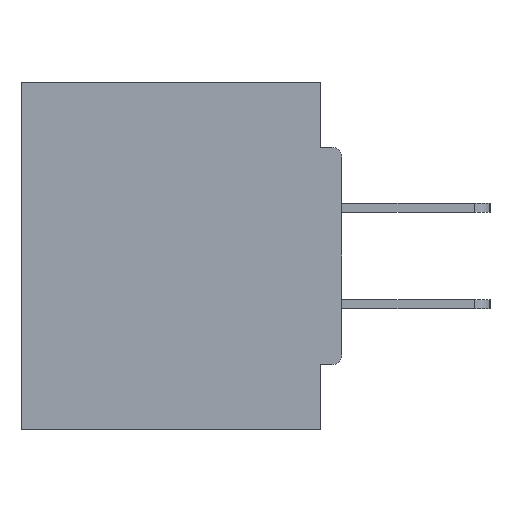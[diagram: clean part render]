
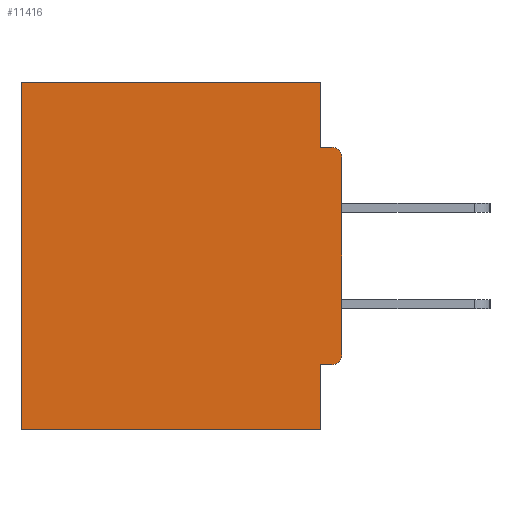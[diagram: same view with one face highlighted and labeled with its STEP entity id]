
A CAD part, left-side view. The second image highlights one B-rep face of the part: STEP entity #11416.
In plain terms, the highlighted planar face has unit normal (-1, 0, 0).
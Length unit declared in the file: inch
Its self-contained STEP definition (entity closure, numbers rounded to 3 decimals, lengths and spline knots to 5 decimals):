
#452 = DIRECTION ( 'NONE',  ( -1., 0., 0. ) ) ;
#820 = CARTESIAN_POINT ( 'NONE',  ( 0.298, 0.031, -0.4065 ) ) ;
#988 = DIRECTION ( 'NONE',  ( 0., 0., -1. ) ) ;
#1395 = AXIS2_PLACEMENT_3D ( 'NONE', #8110, #39183, #17584 ) ;
#1457 = VECTOR ( 'NONE', #15392, 39.37008 ) ;
#1541 = CARTESIAN_POINT ( 'NONE',  ( 0.298, 0.015, -0.4065 ) ) ;
#2151 = DIRECTION ( 'NONE',  ( 0., 0., -1. ) ) ;
#2194 = VERTEX_POINT ( 'NONE', #28801 ) ;
#2297 = LINE ( 'NONE', #12856, #6723 ) ;
#2359 = ORIENTED_EDGE ( 'NONE', *, *, #25466, .F. ) ;
#4178 = DIRECTION ( 'NONE',  ( 0., -1., 0. ) ) ;
#4212 = DIRECTION ( 'NONE',  ( 0., 0., -1. ) ) ;
#4924 = VECTOR ( 'NONE', #21846, 39.37008 ) ;
#5265 = ORIENTED_EDGE ( 'NONE', *, *, #29698, .T. ) ;
#5344 = CARTESIAN_POINT ( 'NONE',  ( 0.298, 0.031, 0. ) ) ;
#6353 = VERTEX_POINT ( 'NONE', #1541 ) ;
#6672 = VERTEX_POINT ( 'NONE', #12775 ) ;
#6723 = VECTOR ( 'NONE', #15697, 39.37008 ) ;
#6793 = LINE ( 'NONE', #25737, #36395 ) ;
#7207 = LINE ( 'NONE', #35267, #36298 ) ;
#7228 = EDGE_CURVE ( 'NONE', #10068, #6672, #9924, .T. ) ;
#8110 = CARTESIAN_POINT ( 'NONE',  ( 0.298, 0., 0. ) ) ;
#8902 = CARTESIAN_POINT ( 'NONE',  ( 0.298, 0., -0.5 ) ) ;
#8995 = EDGE_CURVE ( 'NONE', #6353, #25177, #26716, .T. ) ;
#9034 = DIRECTION ( 'NONE',  ( 0., 1., 0. ) ) ;
#9660 = CARTESIAN_POINT ( 'NONE',  ( 0.298, 0.031, -0.0935 ) ) ;
#9924 = LINE ( 'NONE', #25129, #39048 ) ;
#10068 = VERTEX_POINT ( 'NONE', #5344 ) ;
#10273 = CARTESIAN_POINT ( 'NONE',  ( 0.298, 0.015, -0.0935 ) ) ;
#10296 = VERTEX_POINT ( 'NONE', #820 ) ;
#10575 = CARTESIAN_POINT ( 'NONE',  ( 0.298, 0., -0.0935 ) ) ;
#11249 = VERTEX_POINT ( 'NONE', #35644 ) ;
#11416 = ADVANCED_FACE ( 'NONE', ( #39163 ), #29515, .F. ) ;
#12499 = CARTESIAN_POINT ( 'NONE',  ( 0.298, 0., 0. ) ) ;
#12775 = CARTESIAN_POINT ( 'NONE',  ( 0.298, 0.46, 0. ) ) ;
#12856 = CARTESIAN_POINT ( 'NONE',  ( 0.298, 0.031, -0.5 ) ) ;
#12966 = CARTESIAN_POINT ( 'NONE',  ( 0.298, 0.015, -0.3915 ) ) ;
#14225 = ORIENTED_EDGE ( 'NONE', *, *, #31308, .F. ) ;
#14509 = ORIENTED_EDGE ( 'NONE', *, *, #17757, .T. ) ;
#15040 = AXIS2_PLACEMENT_3D ( 'NONE', #30118, #33090, #2151 ) ;
#15070 = LINE ( 'NONE', #27434, #1457 ) ;
#15392 = DIRECTION ( 'NONE',  ( 0., 1., 0. ) ) ;
#15697 = DIRECTION ( 'NONE',  ( 0., 0., -1. ) ) ;
#16772 = ORIENTED_EDGE ( 'NONE', *, *, #24386, .F. ) ;
#16937 = LINE ( 'NONE', #8902, #22774 ) ;
#17584 = DIRECTION ( 'NONE',  ( 0., 0., -1. ) ) ;
#17757 = EDGE_CURVE ( 'NONE', #6672, #36067, #7207, .T. ) ;
#18346 = VERTEX_POINT ( 'NONE', #10273 ) ;
#21399 = LINE ( 'NONE', #12499, #4924 ) ;
#21846 = DIRECTION ( 'NONE',  ( 0., 0., -1. ) ) ;
#22373 = DIRECTION ( 'NONE',  ( 0., 0., -1. ) ) ;
#22774 = VECTOR ( 'NONE', #9034, 39.37008 ) ;
#22905 = CIRCLE ( 'NONE', #15040, 0.015 ) ;
#23426 = CARTESIAN_POINT ( 'NONE',  ( 0.298, 0., -0.3915 ) ) ;
#24315 = VERTEX_POINT ( 'NONE', #9660 ) ;
#24386 = EDGE_CURVE ( 'NONE', #11249, #25177, #21399, .T. ) ;
#25039 = ORIENTED_EDGE ( 'NONE', *, *, #36988, .F. ) ;
#25129 = CARTESIAN_POINT ( 'NONE',  ( 0.298, 0., 0. ) ) ;
#25177 = VERTEX_POINT ( 'NONE', #23426 ) ;
#25466 = EDGE_CURVE ( 'NONE', #2194, #36067, #16937, .T. ) ;
#25737 = CARTESIAN_POINT ( 'NONE',  ( 0.298, 0.031, -0.5 ) ) ;
#26505 = AXIS2_PLACEMENT_3D ( 'NONE', #12966, #452, #988 ) ;
#26621 = CARTESIAN_POINT ( 'NONE',  ( 0.298, 0.46, -0.5 ) ) ;
#26716 = CIRCLE ( 'NONE', #26505, 0.015 ) ;
#27434 = CARTESIAN_POINT ( 'NONE',  ( 0.298, 0., -0.4065 ) ) ;
#28212 = ORIENTED_EDGE ( 'NONE', *, *, #34033, .F. ) ;
#28801 = CARTESIAN_POINT ( 'NONE',  ( 0.298, 0.031, -0.5 ) ) ;
#29515 = PLANE ( 'NONE',  #1395 ) ;
#29653 = ORIENTED_EDGE ( 'NONE', *, *, #8995, .T. ) ;
#29698 = EDGE_CURVE ( 'NONE', #11249, #18346, #22905, .T. ) ;
#30118 = CARTESIAN_POINT ( 'NONE',  ( 0.298, 0.015, -0.1085 ) ) ;
#31308 = EDGE_CURVE ( 'NONE', #10068, #24315, #2297, .T. ) ;
#32775 = VECTOR ( 'NONE', #4178, 39.37008 ) ;
#33090 = DIRECTION ( 'NONE',  ( -1., 0., 0. ) ) ;
#34033 = EDGE_CURVE ( 'NONE', #24315, #18346, #36197, .T. ) ;
#34641 = EDGE_LOOP ( 'NONE', ( #5265, #28212, #14225, #38673, #14509, #2359, #39681, #25039, #29653, #16772 ) ) ;
#35267 = CARTESIAN_POINT ( 'NONE',  ( 0.298, 0.46, 0. ) ) ;
#35644 = CARTESIAN_POINT ( 'NONE',  ( 0.298, 0., -0.1085 ) ) ;
#36067 = VERTEX_POINT ( 'NONE', #26621 ) ;
#36197 = LINE ( 'NONE', #10575, #32775 ) ;
#36298 = VECTOR ( 'NONE', #4212, 39.37008 ) ;
#36395 = VECTOR ( 'NONE', #22373, 39.37008 ) ;
#36988 = EDGE_CURVE ( 'NONE', #6353, #10296, #15070, .T. ) ;
#37684 = DIRECTION ( 'NONE',  ( 0., 1., 0. ) ) ;
#37914 = EDGE_CURVE ( 'NONE', #10296, #2194, #6793, .T. ) ;
#38673 = ORIENTED_EDGE ( 'NONE', *, *, #7228, .T. ) ;
#39048 = VECTOR ( 'NONE', #37684, 39.37008 ) ;
#39163 = FACE_OUTER_BOUND ( 'NONE', #34641, .T. ) ;
#39183 = DIRECTION ( 'NONE',  ( 1., 0., 0. ) ) ;
#39681 = ORIENTED_EDGE ( 'NONE', *, *, #37914, .F. ) ;
